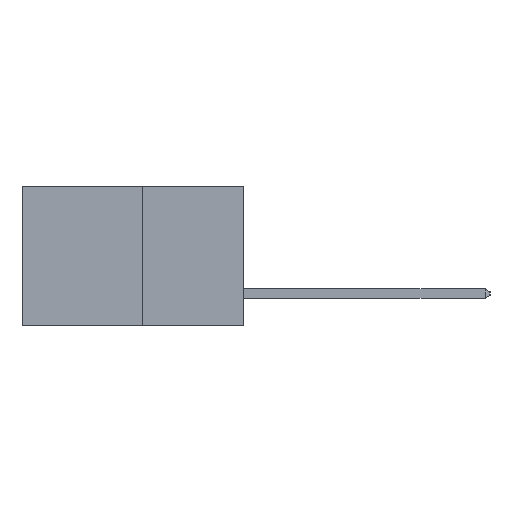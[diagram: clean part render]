
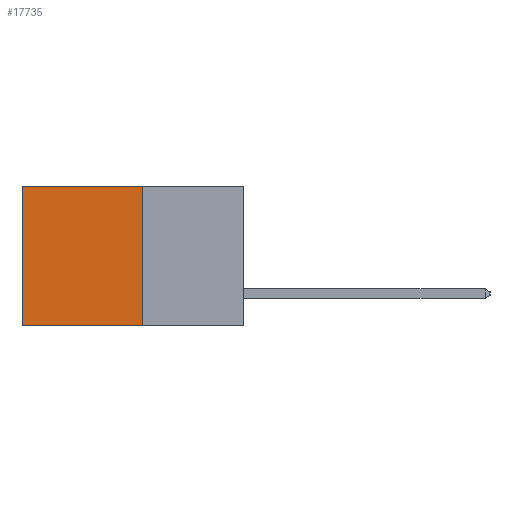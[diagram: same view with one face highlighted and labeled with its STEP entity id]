
A CAD part, left-side view. The second image highlights one B-rep face of the part: STEP entity #17735.
In plain terms, the highlighted planar face has unit normal (-1, 0, 0).
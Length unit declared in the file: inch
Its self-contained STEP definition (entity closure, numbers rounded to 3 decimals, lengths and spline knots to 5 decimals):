
#463 = CARTESIAN_POINT ( 'NONE',  ( 0.277, 0.59, -0.37 ) ) ;
#1285 = EDGE_CURVE ( 'NONE', #15626, #8237, #13108, .T. ) ;
#1425 = ORIENTED_EDGE ( 'NONE', *, *, #6930, .T. ) ;
#1616 = VECTOR ( 'NONE', #8760, 39.37008 ) ;
#2111 = LINE ( 'NONE', #8863, #1616 ) ;
#3575 = VECTOR ( 'NONE', #10279, 39.37008 ) ;
#4779 = ORIENTED_EDGE ( 'NONE', *, *, #1285, .F. ) ;
#5189 = FACE_OUTER_BOUND ( 'NONE', #14185, .T. ) ;
#5461 = DIRECTION ( 'NONE',  ( 1., 0., 0. ) ) ;
#6767 = VECTOR ( 'NONE', #12427, 39.37008 ) ;
#6839 = EDGE_CURVE ( 'NONE', #8237, #8333, #7598, .T. ) ;
#6914 = CARTESIAN_POINT ( 'NONE',  ( 0.277, 0.27, -0.37 ) ) ;
#6930 = EDGE_CURVE ( 'NONE', #15626, #7461, #2111, .T. ) ;
#7132 = CARTESIAN_POINT ( 'NONE',  ( 0.277, 0.59, 0. ) ) ;
#7461 = VERTEX_POINT ( 'NONE', #7132 ) ;
#7535 = ORIENTED_EDGE ( 'NONE', *, *, #6839, .F. ) ;
#7598 = LINE ( 'NONE', #10308, #3575 ) ;
#8173 = ORIENTED_EDGE ( 'NONE', *, *, #11556, .T. ) ;
#8237 = VERTEX_POINT ( 'NONE', #15976 ) ;
#8333 = VERTEX_POINT ( 'NONE', #13356 ) ;
#8760 = DIRECTION ( 'NONE',  ( 0., 1., 0. ) ) ;
#8863 = CARTESIAN_POINT ( 'NONE',  ( 0.277, 0.27, 0. ) ) ;
#8891 = VECTOR ( 'NONE', #11959, 39.37008 ) ;
#10279 = DIRECTION ( 'NONE',  ( 0., 1., 0. ) ) ;
#10308 = CARTESIAN_POINT ( 'NONE',  ( 0.277, 0.27, -0.37 ) ) ;
#11556 = EDGE_CURVE ( 'NONE', #7461, #8333, #14410, .T. ) ;
#11959 = DIRECTION ( 'NONE',  ( 0., 0., -1. ) ) ;
#12035 = CARTESIAN_POINT ( 'NONE',  ( 0.277, 0.27, -0.37 ) ) ;
#12427 = DIRECTION ( 'NONE',  ( 0., 0., -1. ) ) ;
#12709 = PLANE ( 'NONE',  #15146 ) ;
#13108 = LINE ( 'NONE', #12035, #8891 ) ;
#13356 = CARTESIAN_POINT ( 'NONE',  ( 0.277, 0.59, -0.37 ) ) ;
#14185 = EDGE_LOOP ( 'NONE', ( #8173, #7535, #4779, #1425 ) ) ;
#14410 = LINE ( 'NONE', #463, #6767 ) ;
#15146 = AXIS2_PLACEMENT_3D ( 'NONE', #6914, #5461, #15597 ) ;
#15597 = DIRECTION ( 'NONE',  ( 0., 0., -1. ) ) ;
#15626 = VERTEX_POINT ( 'NONE', #17444 ) ;
#15976 = CARTESIAN_POINT ( 'NONE',  ( 0.277, 0.27, -0.37 ) ) ;
#17444 = CARTESIAN_POINT ( 'NONE',  ( 0.277, 0.27, 0. ) ) ;
#17735 = ADVANCED_FACE ( 'NONE', ( #5189 ), #12709, .F. ) ;
